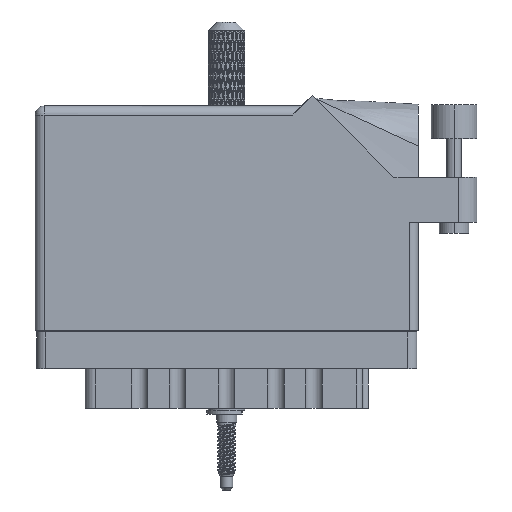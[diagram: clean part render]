
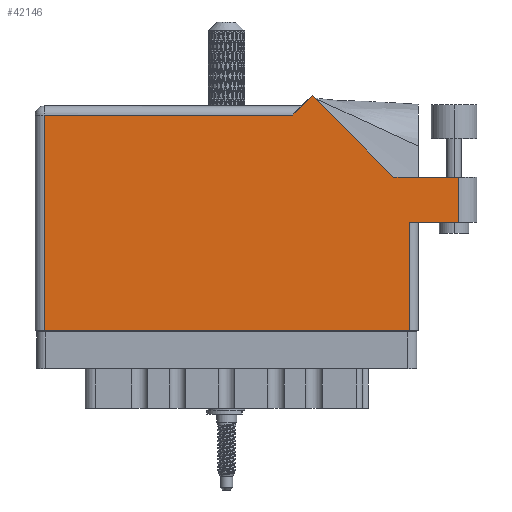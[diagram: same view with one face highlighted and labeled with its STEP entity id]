
A CAD part, front view. The second image highlights one B-rep face of the part: STEP entity #42146.
In plain terms, the highlighted face is planar.
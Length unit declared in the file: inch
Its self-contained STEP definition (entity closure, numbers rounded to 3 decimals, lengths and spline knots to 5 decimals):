
#206 = LINE ( 'NONE', #28610, #32189 ) ;
#1059 = VECTOR ( 'NONE', #59886, 39.37008 ) ;
#1259 = LINE ( 'NONE', #93636, #26772 ) ;
#1572 = LINE ( 'NONE', #29962, #27252 ) ;
#1613 = VERTEX_POINT ( 'NONE', #106723 ) ;
#8682 = CARTESIAN_POINT ( 'NONE',  ( 1.88971, 1.60071, 0. ) ) ;
#10072 = EDGE_CURVE ( 'NONE', #74519, #57903, #52780, .T. ) ;
#11803 = VECTOR ( 'NONE', #74431, 39.37008 ) ;
#16540 = ORIENTED_EDGE ( 'NONE', *, *, #116992, .T. ) ;
#17152 = EDGE_LOOP ( 'NONE', ( #16540, #50124, #80136, #39457, #59321, #46844, #89293, #71978, #97610 ) ) ;
#20902 = DIRECTION ( 'NONE',  ( 1., 0., 0. ) ) ;
#24055 = AXIS2_PLACEMENT_3D ( 'NONE', #55636, #27283, #74349 ) ;
#25351 = VERTEX_POINT ( 'NONE', #58852 ) ;
#26772 = VECTOR ( 'NONE', #74911, 39.37008 ) ;
#27252 = VECTOR ( 'NONE', #20902, 39.37008 ) ;
#27280 = VERTEX_POINT ( 'NONE', #97843 ) ;
#27283 = DIRECTION ( 'NONE',  ( 0., 0., -1. ) ) ;
#28478 = PLANE ( 'NONE',  #24055 ) ;
#28610 = CARTESIAN_POINT ( 'NONE',  ( 3.012, 1.044, 0. ) ) ;
#29962 = CARTESIAN_POINT ( 'NONE',  ( 2.612, 0.737, 0. ) ) ;
#32189 = VECTOR ( 'NONE', #101052, 39.37008 ) ;
#36945 = EDGE_CURVE ( 'NONE', #78716, #94410, #43974, .T. ) ;
#39457 = ORIENTED_EDGE ( 'NONE', *, *, #36945, .T. ) ;
#41371 = LINE ( 'NONE', #114420, #102494 ) ;
#42146 = ADVANCED_FACE ( 'NONE', ( #111194 ), #28478, .F. ) ;
#43974 = LINE ( 'NONE', #80766, #102569 ) ;
#46844 = ORIENTED_EDGE ( 'NONE', *, *, #10072, .T. ) ;
#50124 = ORIENTED_EDGE ( 'NONE', *, *, #58795, .T. ) ;
#50347 = VECTOR ( 'NONE', #93320, 39.37008 ) ;
#52780 = LINE ( 'NONE', #108294, #98007 ) ;
#55152 = CARTESIAN_POINT ( 'NONE',  ( 1.819, 1.53, 0. ) ) ;
#55225 = CARTESIAN_POINT ( 'NONE',  ( 2.55, 0., 0. ) ) ;
#55636 = CARTESIAN_POINT ( 'NONE',  ( 0., 1.53, 0. ) ) ;
#56889 = EDGE_CURVE ( 'NONE', #57903, #27280, #1259, .T. ) ;
#56911 = LINE ( 'NONE', #55152, #11803 ) ;
#57089 = DIRECTION ( 'NONE',  ( 0., 1., 0. ) ) ;
#57903 = VERTEX_POINT ( 'NONE', #94304 ) ;
#58795 = EDGE_CURVE ( 'NONE', #65330, #25351, #97880, .T. ) ;
#58852 = CARTESIAN_POINT ( 'NONE',  ( 2.887, 1.044, 0. ) ) ;
#59321 = ORIENTED_EDGE ( 'NONE', *, *, #91072, .T. ) ;
#59886 = DIRECTION ( 'NONE',  ( 0., 1., 0. ) ) ;
#62271 = EDGE_CURVE ( 'NONE', #25351, #78716, #206, .T. ) ;
#65330 = VERTEX_POINT ( 'NONE', #89444 ) ;
#71978 = ORIENTED_EDGE ( 'NONE', *, *, #117752, .T. ) ;
#72330 = DIRECTION ( 'NONE',  ( -0.707, 0.707, 0. ) ) ;
#73423 = CARTESIAN_POINT ( 'NONE',  ( 0., 0., 0. ) ) ;
#74349 = DIRECTION ( 'NONE',  ( -1., 0., 0. ) ) ;
#74431 = DIRECTION ( 'NONE',  ( -0.707, -0.707, 0. ) ) ;
#74519 = VERTEX_POINT ( 'NONE', #94278 ) ;
#74911 = DIRECTION ( 'NONE',  ( 0., -1., 0. ) ) ;
#78716 = VERTEX_POINT ( 'NONE', #92046 ) ;
#80136 = ORIENTED_EDGE ( 'NONE', *, *, #62271, .T. ) ;
#80766 = CARTESIAN_POINT ( 'NONE',  ( 2.44642, 1.044, 0. ) ) ;
#84624 = VERTEX_POINT ( 'NONE', #55225 ) ;
#88833 = CARTESIAN_POINT ( 'NONE',  ( 2.887, 1.044, 0. ) ) ;
#89293 = ORIENTED_EDGE ( 'NONE', *, *, #56889, .T. ) ;
#89444 = CARTESIAN_POINT ( 'NONE',  ( 2.887, 0.737, 0. ) ) ;
#91072 = EDGE_CURVE ( 'NONE', #94410, #74519, #56911, .T. ) ;
#92046 = CARTESIAN_POINT ( 'NONE',  ( 2.44642, 1.044, 0. ) ) ;
#93320 = DIRECTION ( 'NONE',  ( 1., 0., 0. ) ) ;
#93636 = CARTESIAN_POINT ( 'NONE',  ( 0.062, 0., 0. ) ) ;
#94278 = CARTESIAN_POINT ( 'NONE',  ( 1.757, 1.468, 0. ) ) ;
#94304 = CARTESIAN_POINT ( 'NONE',  ( 0.062, 1.468, 0. ) ) ;
#94410 = VERTEX_POINT ( 'NONE', #8682 ) ;
#97610 = ORIENTED_EDGE ( 'NONE', *, *, #114737, .T. ) ;
#97843 = CARTESIAN_POINT ( 'NONE',  ( 0.062, 0., 0. ) ) ;
#97880 = LINE ( 'NONE', #88833, #1059 ) ;
#98007 = VECTOR ( 'NONE', #109482, 39.37008 ) ;
#101052 = DIRECTION ( 'NONE',  ( -1., 0., 0. ) ) ;
#102494 = VECTOR ( 'NONE', #57089, 39.37008 ) ;
#102569 = VECTOR ( 'NONE', #72330, 39.37008 ) ;
#106723 = CARTESIAN_POINT ( 'NONE',  ( 2.55, 0.737, 0. ) ) ;
#108294 = CARTESIAN_POINT ( 'NONE',  ( 0., 1.468, 0. ) ) ;
#109482 = DIRECTION ( 'NONE',  ( -1., 0., 0. ) ) ;
#111194 = FACE_OUTER_BOUND ( 'NONE', #17152, .T. ) ;
#114420 = CARTESIAN_POINT ( 'NONE',  ( 2.55, 0.737, 0. ) ) ;
#114737 = EDGE_CURVE ( 'NONE', #84624, #1613, #41371, .T. ) ;
#116992 = EDGE_CURVE ( 'NONE', #1613, #65330, #1572, .T. ) ;
#117516 = LINE ( 'NONE', #73423, #50347 ) ;
#117752 = EDGE_CURVE ( 'NONE', #27280, #84624, #117516, .T. ) ;
